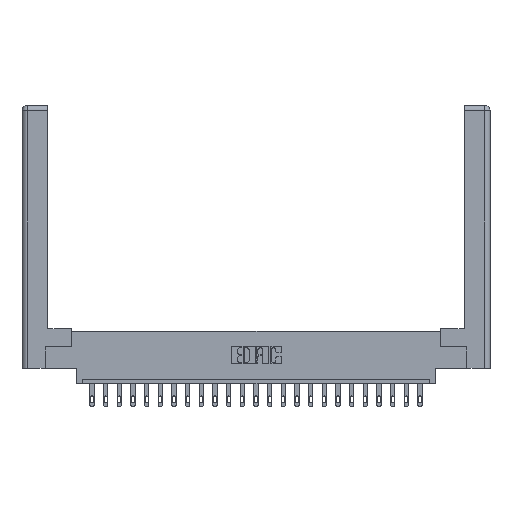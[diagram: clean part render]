
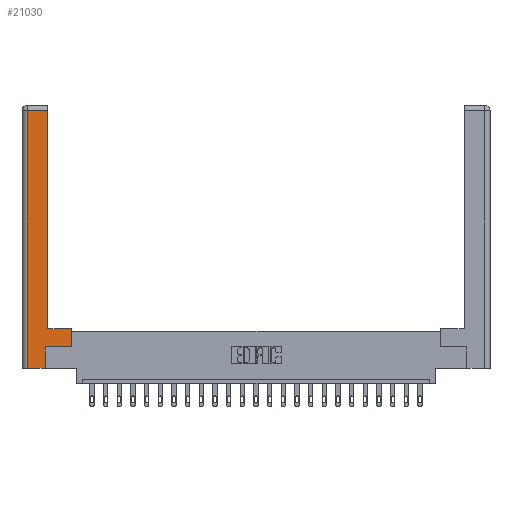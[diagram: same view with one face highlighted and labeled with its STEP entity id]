
A CAD part, top view. The second image highlights one B-rep face of the part: STEP entity #21030.
In plain terms, the highlighted planar face has unit normal (0, 0, 1).
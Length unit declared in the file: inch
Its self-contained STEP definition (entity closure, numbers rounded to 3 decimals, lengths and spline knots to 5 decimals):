
#141 = LINE ( 'NONE', #14851, #14941 ) ;
#361 = FACE_OUTER_BOUND ( 'NONE', #6428, .T. ) ;
#781 = CARTESIAN_POINT ( 'NONE',  ( 0.295, 0.45, 0. ) ) ;
#2197 = LINE ( 'NONE', #16842, #12390 ) ;
#3344 = CARTESIAN_POINT ( 'NONE',  ( 0.0615, 0., 0. ) ) ;
#4181 = LINE ( 'NONE', #8142, #17794 ) ;
#4594 = CARTESIAN_POINT ( 'NONE',  ( 0.265, 0.245, 0. ) ) ;
#4939 = DIRECTION ( 'NONE',  ( -1., 0., 0. ) ) ;
#5290 = VERTEX_POINT ( 'NONE', #9390 ) ;
#5448 = CARTESIAN_POINT ( 'NONE',  ( 0.265, 0., 0. ) ) ;
#5715 = CARTESIAN_POINT ( 'NONE',  ( 0.0615, 2.94, 0. ) ) ;
#6210 = EDGE_CURVE ( 'NONE', #13231, #20115, #19616, .T. ) ;
#6259 = DIRECTION ( 'NONE',  ( -1., 0., 0. ) ) ;
#6368 = DIRECTION ( 'NONE',  ( 0., 1., 0. ) ) ;
#6428 = EDGE_LOOP ( 'NONE', ( #17154, #9781, #12756, #22677, #6520, #14420, #16222, #13841 ) ) ;
#6510 = VERTEX_POINT ( 'NONE', #13521 ) ;
#6520 = ORIENTED_EDGE ( 'NONE', *, *, #11145, .T. ) ;
#7719 = VECTOR ( 'NONE', #13563, 39.37008 ) ;
#7772 = VERTEX_POINT ( 'NONE', #18753 ) ;
#8109 = CARTESIAN_POINT ( 'NONE',  ( 0.565, 0.45, 0. ) ) ;
#8142 = CARTESIAN_POINT ( 'NONE',  ( 0.0615, 2.94, 0. ) ) ;
#8319 = EDGE_CURVE ( 'NONE', #7772, #9559, #9236, .T. ) ;
#9236 = LINE ( 'NONE', #16232, #9808 ) ;
#9390 = CARTESIAN_POINT ( 'NONE',  ( 0.565, 0.45, 0. ) ) ;
#9559 = VERTEX_POINT ( 'NONE', #5448 ) ;
#9781 = ORIENTED_EDGE ( 'NONE', *, *, #16674, .T. ) ;
#9808 = VECTOR ( 'NONE', #18097, 39.37008 ) ;
#9951 = VERTEX_POINT ( 'NONE', #5715 ) ;
#11145 = EDGE_CURVE ( 'NONE', #9559, #13231, #2197, .T. ) ;
#11767 = CARTESIAN_POINT ( 'NONE',  ( 0.295, 2.94, 0. ) ) ;
#11831 = DIRECTION ( 'NONE',  ( 0., -1., 0. ) ) ;
#11843 = LINE ( 'NONE', #8109, #18922 ) ;
#12153 = EDGE_CURVE ( 'NONE', #6510, #15285, #141, .T. ) ;
#12390 = VECTOR ( 'NONE', #6368, 39.37008 ) ;
#12756 = ORIENTED_EDGE ( 'NONE', *, *, #16735, .T. ) ;
#12864 = DIRECTION ( 'NONE',  ( 0., 1., 0. ) ) ;
#13231 = VERTEX_POINT ( 'NONE', #4594 ) ;
#13351 = DIRECTION ( 'NONE',  ( 0., 1., 0. ) ) ;
#13447 = VECTOR ( 'NONE', #11831, 39.37008 ) ;
#13521 = CARTESIAN_POINT ( 'NONE',  ( 0.295, 0.45, 0. ) ) ;
#13563 = DIRECTION ( 'NONE',  ( 1., 0., 0. ) ) ;
#13836 = VECTOR ( 'NONE', #6259, 39.37008 ) ;
#13841 = ORIENTED_EDGE ( 'NONE', *, *, #19410, .T. ) ;
#14420 = ORIENTED_EDGE ( 'NONE', *, *, #6210, .T. ) ;
#14851 = CARTESIAN_POINT ( 'NONE',  ( 0.295, 3., 0. ) ) ;
#14941 = VECTOR ( 'NONE', #12864, 39.37008 ) ;
#15285 = VERTEX_POINT ( 'NONE', #11767 ) ;
#16222 = ORIENTED_EDGE ( 'NONE', *, *, #19366, .T. ) ;
#16232 = CARTESIAN_POINT ( 'NONE',  ( 0.265, 0., 0. ) ) ;
#16674 = EDGE_CURVE ( 'NONE', #15285, #9951, #4181, .T. ) ;
#16735 = EDGE_CURVE ( 'NONE', #9951, #7772, #20794, .T. ) ;
#16842 = CARTESIAN_POINT ( 'NONE',  ( 0.265, 0.245, 0. ) ) ;
#17154 = ORIENTED_EDGE ( 'NONE', *, *, #12153, .T. ) ;
#17784 = LINE ( 'NONE', #781, #13836 ) ;
#17794 = VECTOR ( 'NONE', #4939, 39.37008 ) ;
#18097 = DIRECTION ( 'NONE',  ( 1., 0., 0. ) ) ;
#18753 = CARTESIAN_POINT ( 'NONE',  ( 0.0615, 0., 0. ) ) ;
#18922 = VECTOR ( 'NONE', #13351, 39.37008 ) ;
#19366 = EDGE_CURVE ( 'NONE', #20115, #5290, #11843, .T. ) ;
#19410 = EDGE_CURVE ( 'NONE', #5290, #6510, #17784, .T. ) ;
#19616 = LINE ( 'NONE', #22548, #7719 ) ;
#20115 = VERTEX_POINT ( 'NONE', #21515 ) ;
#20794 = LINE ( 'NONE', #3344, #13447 ) ;
#21030 = ADVANCED_FACE ( 'NONE', ( #361 ), #23416, .F. ) ;
#21444 = CARTESIAN_POINT ( 'NONE',  ( 0., 0., 0. ) ) ;
#21515 = CARTESIAN_POINT ( 'NONE',  ( 0.565, 0.245, 0. ) ) ;
#21598 = DIRECTION ( 'NONE',  ( 0., 0., -1. ) ) ;
#22548 = CARTESIAN_POINT ( 'NONE',  ( 0.565, 0.245, 0. ) ) ;
#22677 = ORIENTED_EDGE ( 'NONE', *, *, #8319, .T. ) ;
#23090 = AXIS2_PLACEMENT_3D ( 'NONE', #21444, #21598, #23496 ) ;
#23416 = PLANE ( 'NONE',  #23090 ) ;
#23496 = DIRECTION ( 'NONE',  ( -1., 0., 0. ) ) ;
